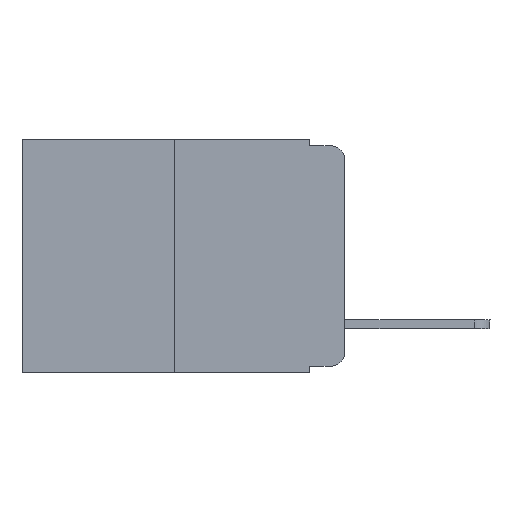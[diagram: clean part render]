
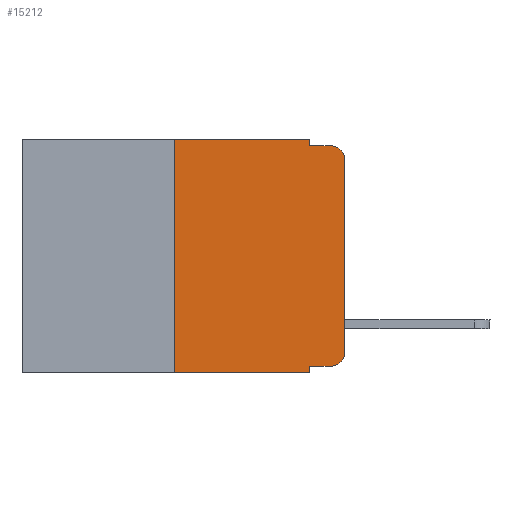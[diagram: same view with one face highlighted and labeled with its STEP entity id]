
A CAD part, left-side view. The second image highlights one B-rep face of the part: STEP entity #15212.
In plain terms, the highlighted planar face has unit normal (-1, 0, 0).
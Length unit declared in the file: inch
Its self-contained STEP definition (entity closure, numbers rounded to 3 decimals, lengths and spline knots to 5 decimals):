
#57 = CARTESIAN_POINT ( 'NONE',  ( 0., 0.051, 0. ) ) ;
#197 = VERTEX_POINT ( 'NONE', #5394 ) ;
#231 = ORIENTED_EDGE ( 'NONE', *, *, #10892, .T. ) ;
#352 = CIRCLE ( 'NONE', #2581, 0.02 ) ;
#358 = FACE_OUTER_BOUND ( 'NONE', #4553, .T. ) ;
#592 = ORIENTED_EDGE ( 'NONE', *, *, #10163, .F. ) ;
#828 = DIRECTION ( 'NONE',  ( 0., -1., 0. ) ) ;
#1131 = CARTESIAN_POINT ( 'NONE',  ( 0., 0.051, -0.01 ) ) ;
#1135 = ORIENTED_EDGE ( 'NONE', *, *, #5902, .T. ) ;
#1727 = CARTESIAN_POINT ( 'NONE',  ( 0., 0.02, -0.333 ) ) ;
#1768 = PLANE ( 'NONE',  #14536 ) ;
#2202 = VERTEX_POINT ( 'NONE', #16096 ) ;
#2298 = DIRECTION ( 'NONE',  ( -1., 0., 0. ) ) ;
#2353 = DIRECTION ( 'NONE',  ( 0., 0., 1. ) ) ;
#2403 = VECTOR ( 'NONE', #6074, 39.37008 ) ;
#2565 = CARTESIAN_POINT ( 'NONE',  ( 0., 0.051, -0.343 ) ) ;
#2581 = AXIS2_PLACEMENT_3D ( 'NONE', #5738, #11100, #16453 ) ;
#2915 = CARTESIAN_POINT ( 'NONE',  ( 0., 0.473, -0.343 ) ) ;
#3016 = CARTESIAN_POINT ( 'NONE',  ( 0., 0.051, 0. ) ) ;
#3023 = EDGE_CURVE ( 'NONE', #4949, #13466, #4347, .T. ) ;
#3181 = CIRCLE ( 'NONE', #7428, 0.02 ) ;
#3652 = EDGE_CURVE ( 'NONE', #6238, #13810, #352, .T. ) ;
#4252 = LINE ( 'NONE', #2915, #9922 ) ;
#4347 = LINE ( 'NONE', #3016, #6757 ) ;
#4376 = DIRECTION ( 'NONE',  ( 0., -1., 0. ) ) ;
#4381 = VECTOR ( 'NONE', #828, 39.37008 ) ;
#4553 = EDGE_LOOP ( 'NONE', ( #1135, #11808, #13978, #592, #11404, #10769, #5270, #11819, #231, #13418 ) ) ;
#4786 = CARTESIAN_POINT ( 'NONE',  ( 0., 0.473, 0. ) ) ;
#4949 = VERTEX_POINT ( 'NONE', #9244 ) ;
#5013 = LINE ( 'NONE', #15720, #15230 ) ;
#5270 = ORIENTED_EDGE ( 'NONE', *, *, #10852, .T. ) ;
#5394 = CARTESIAN_POINT ( 'NONE',  ( 0., 0.051, -0.01 ) ) ;
#5738 = CARTESIAN_POINT ( 'NONE',  ( 0., 0.02, -0.313 ) ) ;
#5841 = VECTOR ( 'NONE', #13490, 39.37008 ) ;
#5892 = LINE ( 'NONE', #15530, #2403 ) ;
#5902 = EDGE_CURVE ( 'NONE', #13810, #11058, #5013, .T. ) ;
#6074 = DIRECTION ( 'NONE',  ( 0., 0., 1. ) ) ;
#6238 = VERTEX_POINT ( 'NONE', #1727 ) ;
#6455 = CARTESIAN_POINT ( 'NONE',  ( 0., 0., -0.03 ) ) ;
#6508 = LINE ( 'NONE', #1131, #16636 ) ;
#6757 = VECTOR ( 'NONE', #8389, 39.37008 ) ;
#7152 = DIRECTION ( 'NONE',  ( 1., 0., 0. ) ) ;
#7428 = AXIS2_PLACEMENT_3D ( 'NONE', #13194, #2298, #17230 ) ;
#7519 = CARTESIAN_POINT ( 'NONE',  ( 0., 0.051, -0.333 ) ) ;
#8297 = DIRECTION ( 'NONE',  ( 0., -1., 0. ) ) ;
#8389 = DIRECTION ( 'NONE',  ( 0., 0., -1. ) ) ;
#8728 = LINE ( 'NONE', #4786, #4381 ) ;
#9108 = CARTESIAN_POINT ( 'NONE',  ( 0., 0.051, 0. ) ) ;
#9244 = CARTESIAN_POINT ( 'NONE',  ( 0., 0.051, -0.333 ) ) ;
#9922 = VECTOR ( 'NONE', #8297, 39.37008 ) ;
#10147 = CARTESIAN_POINT ( 'NONE',  ( 0., 0.25, -0.343 ) ) ;
#10163 = EDGE_CURVE ( 'NONE', #10214, #197, #10532, .T. ) ;
#10214 = VERTEX_POINT ( 'NONE', #57 ) ;
#10218 = LINE ( 'NONE', #7519, #16138 ) ;
#10532 = LINE ( 'NONE', #9108, #5841 ) ;
#10548 = VERTEX_POINT ( 'NONE', #10147 ) ;
#10769 = ORIENTED_EDGE ( 'NONE', *, *, #13063, .F. ) ;
#10814 = CARTESIAN_POINT ( 'NONE',  ( 0., 0., -0.313 ) ) ;
#10852 = EDGE_CURVE ( 'NONE', #10548, #13466, #4252, .T. ) ;
#10892 = EDGE_CURVE ( 'NONE', #4949, #6238, #10218, .T. ) ;
#11027 = EDGE_CURVE ( 'NONE', #11058, #2202, #3181, .T. ) ;
#11058 = VERTEX_POINT ( 'NONE', #6455 ) ;
#11069 = VERTEX_POINT ( 'NONE', #13020 ) ;
#11100 = DIRECTION ( 'NONE',  ( -1., 0., 0. ) ) ;
#11404 = ORIENTED_EDGE ( 'NONE', *, *, #13274, .F. ) ;
#11808 = ORIENTED_EDGE ( 'NONE', *, *, #11027, .T. ) ;
#11819 = ORIENTED_EDGE ( 'NONE', *, *, #3023, .F. ) ;
#12326 = CARTESIAN_POINT ( 'NONE',  ( 0., 0.473, 0. ) ) ;
#13020 = CARTESIAN_POINT ( 'NONE',  ( 0., 0.25, 0. ) ) ;
#13063 = EDGE_CURVE ( 'NONE', #10548, #11069, #5892, .T. ) ;
#13194 = CARTESIAN_POINT ( 'NONE',  ( 0., 0.02, -0.03 ) ) ;
#13274 = EDGE_CURVE ( 'NONE', #11069, #10214, #8728, .T. ) ;
#13418 = ORIENTED_EDGE ( 'NONE', *, *, #3652, .T. ) ;
#13466 = VERTEX_POINT ( 'NONE', #2565 ) ;
#13490 = DIRECTION ( 'NONE',  ( 0., 0., -1. ) ) ;
#13810 = VERTEX_POINT ( 'NONE', #10814 ) ;
#13891 = DIRECTION ( 'NONE',  ( 0., 0., -1. ) ) ;
#13906 = DIRECTION ( 'NONE',  ( 0., -1., 0. ) ) ;
#13978 = ORIENTED_EDGE ( 'NONE', *, *, #17335, .F. ) ;
#14536 = AXIS2_PLACEMENT_3D ( 'NONE', #12326, #7152, #13891 ) ;
#15212 = ADVANCED_FACE ( 'NONE', ( #358 ), #1768, .F. ) ;
#15230 = VECTOR ( 'NONE', #2353, 39.37008 ) ;
#15530 = CARTESIAN_POINT ( 'NONE',  ( 0., 0.25, 0. ) ) ;
#15720 = CARTESIAN_POINT ( 'NONE',  ( 0., 0., 0. ) ) ;
#16096 = CARTESIAN_POINT ( 'NONE',  ( 0., 0.02, -0.01 ) ) ;
#16138 = VECTOR ( 'NONE', #13906, 39.37008 ) ;
#16453 = DIRECTION ( 'NONE',  ( 0., 0., -1. ) ) ;
#16636 = VECTOR ( 'NONE', #4376, 39.37008 ) ;
#17230 = DIRECTION ( 'NONE',  ( 0., 0., -1. ) ) ;
#17335 = EDGE_CURVE ( 'NONE', #197, #2202, #6508, .T. ) ;
